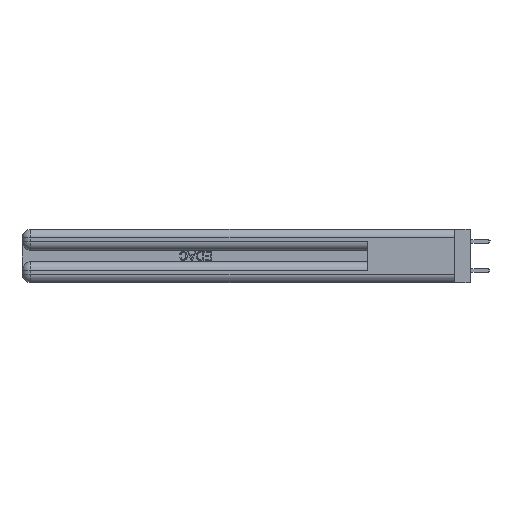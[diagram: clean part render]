
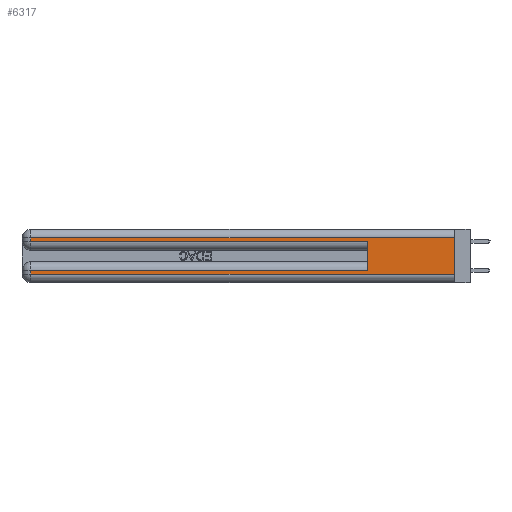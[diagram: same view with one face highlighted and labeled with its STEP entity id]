
A CAD part, left-side view. The second image highlights one B-rep face of the part: STEP entity #6317.
In plain terms, the highlighted planar face has unit normal (-1, 0, 0).
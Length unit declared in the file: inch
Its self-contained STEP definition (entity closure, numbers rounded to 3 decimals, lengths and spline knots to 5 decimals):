
#671 = VECTOR ( 'NONE', #14045, 39.37008 ) ;
#1457 = CARTESIAN_POINT ( 'NONE',  ( 0., 2.94, 0.285 ) ) ;
#2026 = EDGE_CURVE ( 'NONE', #10265, #4634, #8702, .T. ) ;
#2114 = ORIENTED_EDGE ( 'NONE', *, *, #17068, .T. ) ;
#2660 = CARTESIAN_POINT ( 'NONE',  ( 0., 0., 0.06 ) ) ;
#2852 = ORIENTED_EDGE ( 'NONE', *, *, #5870, .F. ) ;
#3050 = VERTEX_POINT ( 'NONE', #10484 ) ;
#3565 = CARTESIAN_POINT ( 'NONE',  ( 0., 0.6, 0.285 ) ) ;
#4546 = ORIENTED_EDGE ( 'NONE', *, *, #25615, .T. ) ;
#4634 = VERTEX_POINT ( 'NONE', #1457 ) ;
#4739 = VECTOR ( 'NONE', #34628, 39.37008 ) ;
#4776 = VECTOR ( 'NONE', #20602, 39.37008 ) ;
#5175 = CARTESIAN_POINT ( 'NONE',  ( 0., 2.94, 0.085 ) ) ;
#5455 = CARTESIAN_POINT ( 'NONE',  ( 0., 2.94, 0.31 ) ) ;
#5870 = EDGE_CURVE ( 'NONE', #39763, #42776, #10028, .T. ) ;
#6017 = VERTEX_POINT ( 'NONE', #25441 ) ;
#6139 = EDGE_CURVE ( 'NONE', #3050, #22848, #35280, .T. ) ;
#6317 = ADVANCED_FACE ( 'NONE', ( #20447 ), #38020, .F. ) ;
#8702 = LINE ( 'NONE', #14060, #35605 ) ;
#10028 = LINE ( 'NONE', #38640, #671 ) ;
#10265 = VERTEX_POINT ( 'NONE', #5455 ) ;
#10484 = CARTESIAN_POINT ( 'NONE',  ( 0., 0.6, 0.085 ) ) ;
#10670 = DIRECTION ( 'NONE',  ( 0., 0., -1. ) ) ;
#12983 = LINE ( 'NONE', #13587, #4739 ) ;
#13435 = ORIENTED_EDGE ( 'NONE', *, *, #6139, .T. ) ;
#13587 = CARTESIAN_POINT ( 'NONE',  ( 0., 0., 0.31 ) ) ;
#14045 = DIRECTION ( 'NONE',  ( 0., 0., -1. ) ) ;
#14057 = EDGE_CURVE ( 'NONE', #6017, #42776, #22594, .T. ) ;
#14060 = CARTESIAN_POINT ( 'NONE',  ( 0., 2.94, 0.37 ) ) ;
#14748 = LINE ( 'NONE', #43389, #40591 ) ;
#16241 = DIRECTION ( 'NONE',  ( 0., 0., 1. ) ) ;
#16931 = CARTESIAN_POINT ( 'NONE',  ( 0., 0., 0.285 ) ) ;
#16983 = CARTESIAN_POINT ( 'NONE',  ( 0., 0., 0.37 ) ) ;
#17068 = EDGE_CURVE ( 'NONE', #4634, #34652, #23485, .T. ) ;
#17537 = EDGE_LOOP ( 'NONE', ( #2852, #4546, #35334, #2114, #29343, #13435, #35426, #23353 ) ) ;
#20447 = FACE_OUTER_BOUND ( 'NONE', #17537, .T. ) ;
#20497 = DIRECTION ( 'NONE',  ( 0., 0., -1. ) ) ;
#20602 = DIRECTION ( 'NONE',  ( 0., -1., 0. ) ) ;
#20994 = DIRECTION ( 'NONE',  ( 0., -1., 0. ) ) ;
#22200 = CARTESIAN_POINT ( 'NONE',  ( 0., 0., 0.31 ) ) ;
#22409 = DIRECTION ( 'NONE',  ( 0., 0., -1. ) ) ;
#22594 = LINE ( 'NONE', #38513, #30786 ) ;
#22848 = VERTEX_POINT ( 'NONE', #5175 ) ;
#23353 = ORIENTED_EDGE ( 'NONE', *, *, #14057, .T. ) ;
#23485 = LINE ( 'NONE', #16931, #4776 ) ;
#25441 = CARTESIAN_POINT ( 'NONE',  ( 0., 2.94, 0.06 ) ) ;
#25615 = EDGE_CURVE ( 'NONE', #39763, #10265, #12983, .T. ) ;
#25987 = VECTOR ( 'NONE', #26056, 39.37008 ) ;
#26056 = DIRECTION ( 'NONE',  ( 0., 1., 0. ) ) ;
#29343 = ORIENTED_EDGE ( 'NONE', *, *, #34385, .F. ) ;
#30786 = VECTOR ( 'NONE', #20994, 39.37008 ) ;
#33817 = LINE ( 'NONE', #37254, #42041 ) ;
#34385 = EDGE_CURVE ( 'NONE', #3050, #34652, #33817, .T. ) ;
#34628 = DIRECTION ( 'NONE',  ( 0., 1., 0. ) ) ;
#34652 = VERTEX_POINT ( 'NONE', #3565 ) ;
#35280 = LINE ( 'NONE', #36460, #25987 ) ;
#35334 = ORIENTED_EDGE ( 'NONE', *, *, #2026, .T. ) ;
#35426 = ORIENTED_EDGE ( 'NONE', *, *, #37647, .T. ) ;
#35605 = VECTOR ( 'NONE', #10670, 39.37008 ) ;
#36460 = CARTESIAN_POINT ( 'NONE',  ( 0., 0., 0.085 ) ) ;
#37254 = CARTESIAN_POINT ( 'NONE',  ( 0., 0.6, 0.145 ) ) ;
#37647 = EDGE_CURVE ( 'NONE', #22848, #6017, #14748, .T. ) ;
#38020 = PLANE ( 'NONE',  #43391 ) ;
#38513 = CARTESIAN_POINT ( 'NONE',  ( 0., 0., 0.06 ) ) ;
#38640 = CARTESIAN_POINT ( 'NONE',  ( 0., 0., 0.37 ) ) ;
#39763 = VERTEX_POINT ( 'NONE', #22200 ) ;
#40591 = VECTOR ( 'NONE', #22409, 39.37008 ) ;
#41518 = DIRECTION ( 'NONE',  ( 1., 0., 0. ) ) ;
#42041 = VECTOR ( 'NONE', #16241, 39.37008 ) ;
#42776 = VERTEX_POINT ( 'NONE', #2660 ) ;
#43389 = CARTESIAN_POINT ( 'NONE',  ( 0., 2.94, 0.37 ) ) ;
#43391 = AXIS2_PLACEMENT_3D ( 'NONE', #16983, #41518, #20497 ) ;
